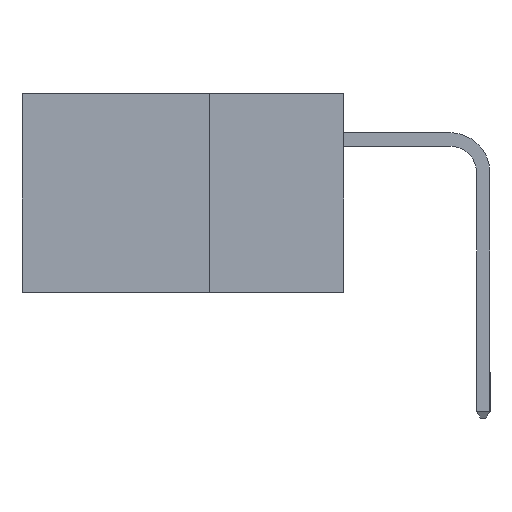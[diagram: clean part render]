
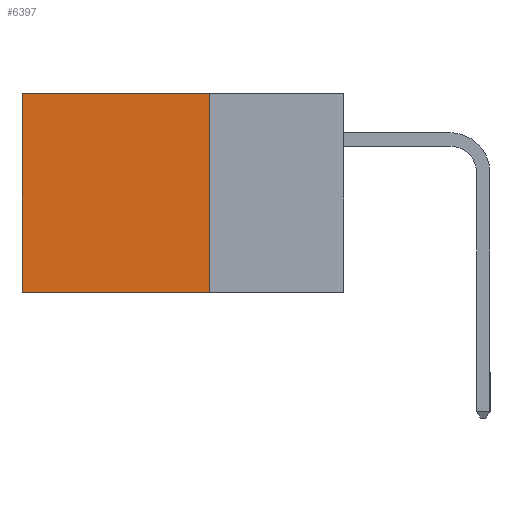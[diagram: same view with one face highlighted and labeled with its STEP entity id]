
A CAD part, left-side view. The second image highlights one B-rep face of the part: STEP entity #6397.
In plain terms, the highlighted planar face has unit normal (-1, 0, 0).
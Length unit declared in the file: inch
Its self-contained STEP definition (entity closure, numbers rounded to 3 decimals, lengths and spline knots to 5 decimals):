
#122 = EDGE_CURVE ( 'NONE', #1634, #4821, #1411, .T. ) ;
#435 = DIRECTION ( 'NONE',  ( 0., 0., -1. ) ) ;
#520 = CARTESIAN_POINT ( 'NONE',  ( 0.298, 0.6, 0. ) ) ;
#976 = CARTESIAN_POINT ( 'NONE',  ( 0.298, 0.25, -0.37 ) ) ;
#1264 = ORIENTED_EDGE ( 'NONE', *, *, #122, .T. ) ;
#1411 = LINE ( 'NONE', #5160, #3332 ) ;
#1486 = CARTESIAN_POINT ( 'NONE',  ( 0.298, 0.25, -0.37 ) ) ;
#1634 = VERTEX_POINT ( 'NONE', #4372 ) ;
#1676 = CARTESIAN_POINT ( 'NONE',  ( 0.298, 0.6, -0.37 ) ) ;
#1941 = EDGE_CURVE ( 'NONE', #5041, #8634, #2461, .T. ) ;
#2041 = PLANE ( 'NONE',  #2525 ) ;
#2461 = LINE ( 'NONE', #1486, #10230 ) ;
#2525 = AXIS2_PLACEMENT_3D ( 'NONE', #5306, #6797, #435 ) ;
#2995 = DIRECTION ( 'NONE',  ( 0., 0., -1. ) ) ;
#3191 = DIRECTION ( 'NONE',  ( 0., 1., 0. ) ) ;
#3332 = VECTOR ( 'NONE', #3609, 39.37008 ) ;
#3609 = DIRECTION ( 'NONE',  ( 0., 1., 0. ) ) ;
#3654 = FACE_OUTER_BOUND ( 'NONE', #5943, .T. ) ;
#4372 = CARTESIAN_POINT ( 'NONE',  ( 0.298, 0.25, 0. ) ) ;
#4821 = VERTEX_POINT ( 'NONE', #5657 ) ;
#4870 = ORIENTED_EDGE ( 'NONE', *, *, #6527, .F. ) ;
#5041 = VERTEX_POINT ( 'NONE', #976 ) ;
#5048 = ORIENTED_EDGE ( 'NONE', *, *, #5887, .T. ) ;
#5160 = CARTESIAN_POINT ( 'NONE',  ( 0.298, 0.25, 0. ) ) ;
#5306 = CARTESIAN_POINT ( 'NONE',  ( 0.298, 0.25, 0. ) ) ;
#5657 = CARTESIAN_POINT ( 'NONE',  ( 0.298, 0.6, 0. ) ) ;
#5887 = EDGE_CURVE ( 'NONE', #4821, #8634, #9802, .T. ) ;
#5940 = VECTOR ( 'NONE', #6967, 39.37008 ) ;
#5943 = EDGE_LOOP ( 'NONE', ( #5048, #6698, #4870, #1264 ) ) ;
#6274 = VECTOR ( 'NONE', #2995, 39.37008 ) ;
#6397 = ADVANCED_FACE ( 'NONE', ( #3654 ), #2041, .F. ) ;
#6527 = EDGE_CURVE ( 'NONE', #1634, #5041, #6971, .T. ) ;
#6698 = ORIENTED_EDGE ( 'NONE', *, *, #1941, .F. ) ;
#6797 = DIRECTION ( 'NONE',  ( 1., 0., 0. ) ) ;
#6967 = DIRECTION ( 'NONE',  ( 0., 0., -1. ) ) ;
#6971 = LINE ( 'NONE', #10313, #5940 ) ;
#8634 = VERTEX_POINT ( 'NONE', #1676 ) ;
#9802 = LINE ( 'NONE', #520, #6274 ) ;
#10230 = VECTOR ( 'NONE', #3191, 39.37008 ) ;
#10313 = CARTESIAN_POINT ( 'NONE',  ( 0.298, 0.25, 0. ) ) ;
